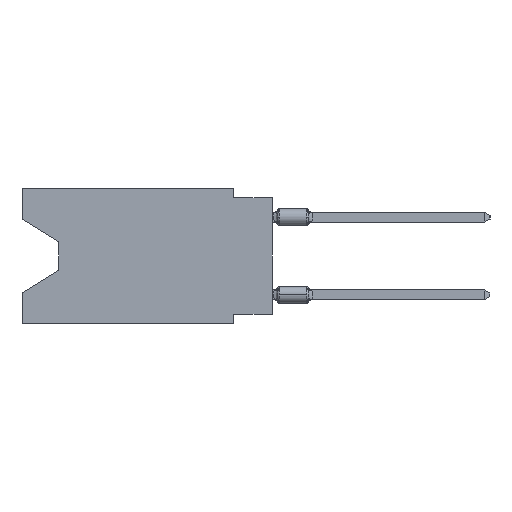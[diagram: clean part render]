
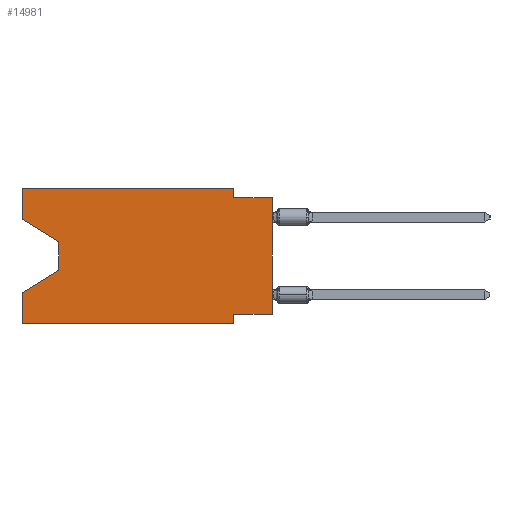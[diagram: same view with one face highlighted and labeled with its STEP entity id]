
A CAD part, left-side view. The second image highlights one B-rep face of the part: STEP entity #14981.
In plain terms, the highlighted planar face has unit normal (-1, 0, 0).
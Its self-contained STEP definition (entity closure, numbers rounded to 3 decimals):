
#58 = EDGE_CURVE ( 'NONE', #21651, #14924, #25264, .T. ) ;
#310 = DIRECTION ( 'NONE',  ( 0., 1., 0. ) ) ;
#496 = VECTOR ( 'NONE', #310, 1000. ) ;
#561 = LINE ( 'NONE', #18892, #3049 ) ;
#662 = DIRECTION ( 'NONE',  ( 0., -0.855, -0.519 ) ) ;
#763 = DIRECTION ( 'NONE',  ( 0., -1., 0. ) ) ;
#778 = CARTESIAN_POINT ( 'NONE',  ( 0., 16.383, -2.038 ) ) ;
#1496 = CARTESIAN_POINT ( 'NONE',  ( 0., 16.383, 0. ) ) ;
#1682 = CARTESIAN_POINT ( 'NONE',  ( 0., 16.383, 0. ) ) ;
#2009 = CARTESIAN_POINT ( 'NONE',  ( 0., 0., -8.255 ) ) ;
#2297 = EDGE_CURVE ( 'NONE', #17027, #20468, #23668, .T. ) ;
#2624 = CARTESIAN_POINT ( 'NONE',  ( 0., 0., -0.635 ) ) ;
#2904 = DIRECTION ( 'NONE',  ( 0., 0., -1. ) ) ;
#2985 = CARTESIAN_POINT ( 'NONE',  ( 0., 2.54, -8.89 ) ) ;
#3049 = VECTOR ( 'NONE', #22472, 1000. ) ;
#3142 = DIRECTION ( 'NONE',  ( 0., -1., 0. ) ) ;
#3189 = LINE ( 'NONE', #19539, #17117 ) ;
#3422 = CARTESIAN_POINT ( 'NONE',  ( 0., 2.54, 0. ) ) ;
#3811 = VECTOR ( 'NONE', #763, 1000. ) ;
#4298 = VECTOR ( 'NONE', #2904, 1000. ) ;
#4360 = VECTOR ( 'NONE', #25423, 1000. ) ;
#5118 = DIRECTION ( 'NONE',  ( 0., 0., 1. ) ) ;
#5386 = EDGE_CURVE ( 'NONE', #6306, #23973, #20982, .T. ) ;
#6306 = VERTEX_POINT ( 'NONE', #17148 ) ;
#6399 = EDGE_LOOP ( 'NONE', ( #22920, #20189, #21703, #6999, #20579, #23457, #20618, #12866, #14134, #13009, #24115, #8139 ) ) ;
#6999 = ORIENTED_EDGE ( 'NONE', *, *, #11934, .F. ) ;
#7342 = LINE ( 'NONE', #1496, #4360 ) ;
#7380 = LINE ( 'NONE', #19235, #26237 ) ;
#7449 = CARTESIAN_POINT ( 'NONE',  ( 0., 2.54, -8.255 ) ) ;
#8139 = ORIENTED_EDGE ( 'NONE', *, *, #11499, .F. ) ;
#9108 = LINE ( 'NONE', #17228, #11582 ) ;
#9348 = CARTESIAN_POINT ( 'NONE',  ( 0., 16.383, -8.89 ) ) ;
#9419 = DIRECTION ( 'NONE',  ( 0., 0., 1. ) ) ;
#9570 = EDGE_CURVE ( 'NONE', #17760, #17027, #22593, .T. ) ;
#9824 = CARTESIAN_POINT ( 'NONE',  ( 0., 16.383, -6.852 ) ) ;
#9869 = CARTESIAN_POINT ( 'NONE',  ( 0., 2.54, 0. ) ) ;
#10535 = EDGE_CURVE ( 'NONE', #17570, #21399, #561, .T. ) ;
#11341 = FACE_OUTER_BOUND ( 'NONE', #6399, .T. ) ;
#11499 = EDGE_CURVE ( 'NONE', #17760, #17570, #7342, .T. ) ;
#11582 = VECTOR ( 'NONE', #3142, 1000. ) ;
#11934 = EDGE_CURVE ( 'NONE', #22085, #24208, #3189, .T. ) ;
#12531 = CARTESIAN_POINT ( 'NONE',  ( 0., 0., -8.255 ) ) ;
#12866 = ORIENTED_EDGE ( 'NONE', *, *, #23775, .T. ) ;
#13009 = ORIENTED_EDGE ( 'NONE', *, *, #19191, .F. ) ;
#13229 = CARTESIAN_POINT ( 'NONE',  ( 0., 16.383, 0. ) ) ;
#14077 = EDGE_CURVE ( 'NONE', #15611, #21651, #14542, .T. ) ;
#14134 = ORIENTED_EDGE ( 'NONE', *, *, #5386, .F. ) ;
#14542 = LINE ( 'NONE', #12531, #496 ) ;
#14862 = AXIS2_PLACEMENT_3D ( 'NONE', #13229, #15606, #19858 ) ;
#14924 = VERTEX_POINT ( 'NONE', #2985 ) ;
#14981 = ADVANCED_FACE ( 'NONE', ( #11341 ), #23333, .F. ) ;
#15606 = DIRECTION ( 'NONE',  ( 1., 0., 0. ) ) ;
#15611 = VERTEX_POINT ( 'NONE', #2009 ) ;
#16270 = CARTESIAN_POINT ( 'NONE',  ( 0., 16.383, -2.038 ) ) ;
#17027 = VERTEX_POINT ( 'NONE', #23278 ) ;
#17117 = VECTOR ( 'NONE', #9419, 1000. ) ;
#17148 = CARTESIAN_POINT ( 'NONE',  ( 0., 2.54, -0.635 ) ) ;
#17228 = CARTESIAN_POINT ( 'NONE',  ( 0., 16.383, -8.89 ) ) ;
#17570 = VERTEX_POINT ( 'NONE', #1682 ) ;
#17595 = LINE ( 'NONE', #21840, #23230 ) ;
#17760 = VERTEX_POINT ( 'NONE', #16270 ) ;
#18892 = CARTESIAN_POINT ( 'NONE',  ( 0., 16.383, 0. ) ) ;
#19191 = EDGE_CURVE ( 'NONE', #21399, #6306, #21631, .T. ) ;
#19235 = CARTESIAN_POINT ( 'NONE',  ( 0., 0., 0. ) ) ;
#19539 = CARTESIAN_POINT ( 'NONE',  ( 0., 16.383, 0. ) ) ;
#19542 = DIRECTION ( 'NONE',  ( 0., 0., -1. ) ) ;
#19632 = EDGE_CURVE ( 'NONE', #22085, #14924, #9108, .T. ) ;
#19684 = CARTESIAN_POINT ( 'NONE',  ( 0., 13.97, -3.505 ) ) ;
#19726 = VECTOR ( 'NONE', #662, 1000. ) ;
#19858 = DIRECTION ( 'NONE',  ( 0., 0., -1. ) ) ;
#20189 = ORIENTED_EDGE ( 'NONE', *, *, #2297, .T. ) ;
#20468 = VERTEX_POINT ( 'NONE', #24039 ) ;
#20481 = VECTOR ( 'NONE', #21118, 1000. ) ;
#20579 = ORIENTED_EDGE ( 'NONE', *, *, #19632, .T. ) ;
#20618 = ORIENTED_EDGE ( 'NONE', *, *, #14077, .F. ) ;
#20982 = LINE ( 'NONE', #2624, #3811 ) ;
#21118 = DIRECTION ( 'NONE',  ( 0., 0., -1. ) ) ;
#21132 = CARTESIAN_POINT ( 'NONE',  ( 0., 2.54, -8.89 ) ) ;
#21399 = VERTEX_POINT ( 'NONE', #9869 ) ;
#21631 = LINE ( 'NONE', #3422, #20481 ) ;
#21651 = VERTEX_POINT ( 'NONE', #7449 ) ;
#21703 = ORIENTED_EDGE ( 'NONE', *, *, #22570, .T. ) ;
#21840 = CARTESIAN_POINT ( 'NONE',  ( 0., 13.97, -5.385 ) ) ;
#21965 = DIRECTION ( 'NONE',  ( 0., 0.855, -0.519 ) ) ;
#22085 = VERTEX_POINT ( 'NONE', #9348 ) ;
#22145 = CARTESIAN_POINT ( 'NONE',  ( 0., 0., -0.635 ) ) ;
#22472 = DIRECTION ( 'NONE',  ( 0., -1., 0. ) ) ;
#22570 = EDGE_CURVE ( 'NONE', #20468, #24208, #17595, .T. ) ;
#22593 = LINE ( 'NONE', #778, #19726 ) ;
#22920 = ORIENTED_EDGE ( 'NONE', *, *, #9570, .T. ) ;
#23230 = VECTOR ( 'NONE', #21965, 1000. ) ;
#23278 = CARTESIAN_POINT ( 'NONE',  ( 0., 13.97, -3.505 ) ) ;
#23333 = PLANE ( 'NONE',  #14862 ) ;
#23457 = ORIENTED_EDGE ( 'NONE', *, *, #58, .F. ) ;
#23668 = LINE ( 'NONE', #19684, #24713 ) ;
#23775 = EDGE_CURVE ( 'NONE', #15611, #23973, #7380, .T. ) ;
#23973 = VERTEX_POINT ( 'NONE', #22145 ) ;
#24039 = CARTESIAN_POINT ( 'NONE',  ( 0., 13.97, -5.385 ) ) ;
#24115 = ORIENTED_EDGE ( 'NONE', *, *, #10535, .F. ) ;
#24208 = VERTEX_POINT ( 'NONE', #9824 ) ;
#24713 = VECTOR ( 'NONE', #19542, 1000. ) ;
#25264 = LINE ( 'NONE', #21132, #4298 ) ;
#25423 = DIRECTION ( 'NONE',  ( 0., 0., 1. ) ) ;
#26237 = VECTOR ( 'NONE', #5118, 1000. ) ;
